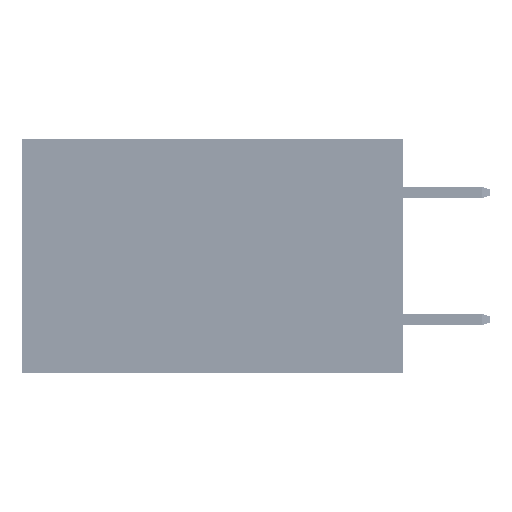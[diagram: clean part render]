
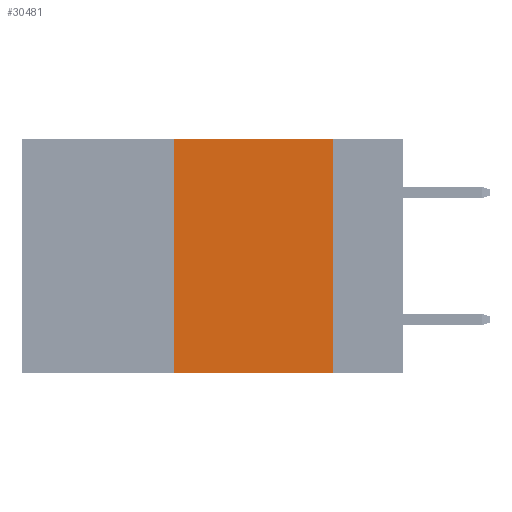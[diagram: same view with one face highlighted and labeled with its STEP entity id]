
A CAD part, left-side view. The second image highlights one B-rep face of the part: STEP entity #30481.
In plain terms, the highlighted planar face has unit normal (-1, 0, 0).
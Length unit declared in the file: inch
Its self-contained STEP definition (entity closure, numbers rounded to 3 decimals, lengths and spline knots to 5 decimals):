
#1029 = ORIENTED_EDGE ( 'NONE', *, *, #42374, .T. ) ;
#2995 = CARTESIAN_POINT ( 'NONE',  ( 0., 0.11, -0.37 ) ) ;
#3222 = DIRECTION ( 'NONE',  ( 0., 0., -1. ) ) ;
#4428 = VECTOR ( 'NONE', #21106, 39.37008 ) ;
#5724 = VECTOR ( 'NONE', #34307, 39.37008 ) ;
#6338 = ORIENTED_EDGE ( 'NONE', *, *, #44842, .F. ) ;
#6445 = VERTEX_POINT ( 'NONE', #46595 ) ;
#6811 = LINE ( 'NONE', #44411, #5724 ) ;
#10175 = EDGE_CURVE ( 'NONE', #6445, #33076, #17138, .T. ) ;
#10407 = CARTESIAN_POINT ( 'NONE',  ( 0., 0.36, 0. ) ) ;
#13045 = VECTOR ( 'NONE', #22034, 39.37008 ) ;
#13066 = AXIS2_PLACEMENT_3D ( 'NONE', #25207, #40283, #3222 ) ;
#13077 = ORIENTED_EDGE ( 'NONE', *, *, #20339, .F. ) ;
#14356 = CARTESIAN_POINT ( 'NONE',  ( 0., 0.36, 0. ) ) ;
#16655 = ORIENTED_EDGE ( 'NONE', *, *, #10175, .F. ) ;
#17138 = LINE ( 'NONE', #14356, #4428 ) ;
#18527 = CARTESIAN_POINT ( 'NONE',  ( 0., 0.11, 0. ) ) ;
#20339 = EDGE_CURVE ( 'NONE', #33916, #28950, #25718, .T. ) ;
#21106 = DIRECTION ( 'NONE',  ( 0., 0., 1. ) ) ;
#21232 = CARTESIAN_POINT ( 'NONE',  ( 0., 0.6, 0. ) ) ;
#21537 = FACE_OUTER_BOUND ( 'NONE', #28124, .T. ) ;
#22034 = DIRECTION ( 'NONE',  ( 0., 0., -1. ) ) ;
#25207 = CARTESIAN_POINT ( 'NONE',  ( 0., 0.6, 0. ) ) ;
#25718 = LINE ( 'NONE', #30183, #13045 ) ;
#28124 = EDGE_LOOP ( 'NONE', ( #13077, #6338, #16655, #1029 ) ) ;
#28950 = VERTEX_POINT ( 'NONE', #2995 ) ;
#29113 = LINE ( 'NONE', #21232, #48536 ) ;
#30183 = CARTESIAN_POINT ( 'NONE',  ( 0., 0.11, 0. ) ) ;
#30481 = ADVANCED_FACE ( 'NONE', ( #21537 ), #36850, .F. ) ;
#32580 = DIRECTION ( 'NONE',  ( 0., -1., 0. ) ) ;
#33076 = VERTEX_POINT ( 'NONE', #10407 ) ;
#33916 = VERTEX_POINT ( 'NONE', #18527 ) ;
#34307 = DIRECTION ( 'NONE',  ( 0., -1., 0. ) ) ;
#36850 = PLANE ( 'NONE',  #13066 ) ;
#40283 = DIRECTION ( 'NONE',  ( 1., 0., 0. ) ) ;
#42374 = EDGE_CURVE ( 'NONE', #6445, #28950, #6811, .T. ) ;
#44411 = CARTESIAN_POINT ( 'NONE',  ( 0., 0.6, -0.37 ) ) ;
#44842 = EDGE_CURVE ( 'NONE', #33076, #33916, #29113, .T. ) ;
#46595 = CARTESIAN_POINT ( 'NONE',  ( 0., 0.36, -0.37 ) ) ;
#48536 = VECTOR ( 'NONE', #32580, 39.37008 ) ;
